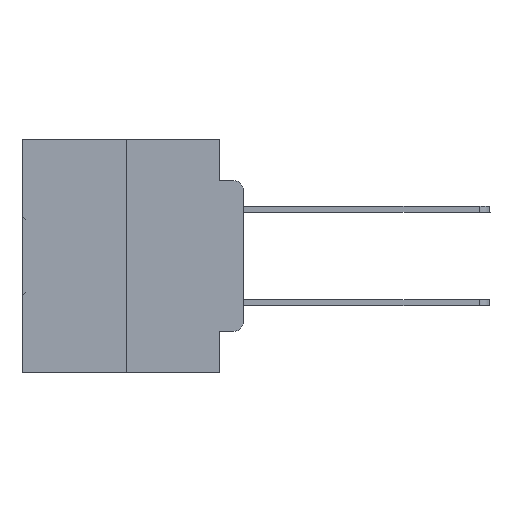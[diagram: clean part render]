
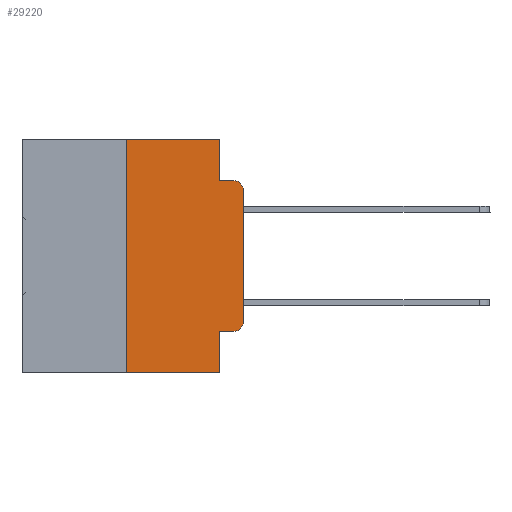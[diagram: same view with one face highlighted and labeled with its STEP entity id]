
A CAD part, left-side view. The second image highlights one B-rep face of the part: STEP entity #29220.
In plain terms, the highlighted planar face has unit normal (-1, 0, 0).
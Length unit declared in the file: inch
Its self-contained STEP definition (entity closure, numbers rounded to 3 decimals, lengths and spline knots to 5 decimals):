
#249 = DIRECTION ( 'NONE',  ( 0., -1., 0. ) ) ;
#351 = ORIENTED_EDGE ( 'NONE', *, *, #30464, .T. ) ;
#605 = AXIS2_PLACEMENT_3D ( 'NONE', #6944, #9692, #12454 ) ;
#1002 = VERTEX_POINT ( 'NONE', #11561 ) ;
#1033 = LINE ( 'NONE', #9492, #12632 ) ;
#1178 = LINE ( 'NONE', #33012, #11439 ) ;
#1340 = DIRECTION ( 'NONE',  ( 0., 0., -1. ) ) ;
#1547 = CARTESIAN_POINT ( 'NONE',  ( 0., 0.051, -0.4115 ) ) ;
#1676 = DIRECTION ( 'NONE',  ( 0., -1., 0. ) ) ;
#2059 = VERTEX_POINT ( 'NONE', #20706 ) ;
#2615 = LINE ( 'NONE', #14983, #34724 ) ;
#2622 = EDGE_CURVE ( 'NONE', #31842, #2059, #31884, .T. ) ;
#2749 = VECTOR ( 'NONE', #5492, 39.37008 ) ;
#3475 = EDGE_CURVE ( 'NONE', #24998, #34093, #28788, .T. ) ;
#4297 = LINE ( 'NONE', #15519, #11556 ) ;
#4590 = ORIENTED_EDGE ( 'NONE', *, *, #22030, .T. ) ;
#4610 = EDGE_CURVE ( 'NONE', #29883, #33204, #4297, .T. ) ;
#4845 = CIRCLE ( 'NONE', #26368, 0.02 ) ;
#4885 = CARTESIAN_POINT ( 'NONE',  ( 0., 0., -0.3915 ) ) ;
#5492 = DIRECTION ( 'NONE',  ( 0., -1., 0. ) ) ;
#6262 = DIRECTION ( 'NONE',  ( -1., 0., 0. ) ) ;
#6421 = LINE ( 'NONE', #1547, #15430 ) ;
#6808 = PLANE ( 'NONE',  #605 ) ;
#6880 = CARTESIAN_POINT ( 'NONE',  ( 0., 0.051, -0.4115 ) ) ;
#6944 = CARTESIAN_POINT ( 'NONE',  ( 0., 0.473, 0. ) ) ;
#7432 = VECTOR ( 'NONE', #32172, 39.37008 ) ;
#8366 = ORIENTED_EDGE ( 'NONE', *, *, #4610, .F. ) ;
#8964 = VERTEX_POINT ( 'NONE', #4885 ) ;
#9171 = EDGE_CURVE ( 'NONE', #1002, #15084, #2615, .T. ) ;
#9340 = AXIS2_PLACEMENT_3D ( 'NONE', #24849, #25208, #13945 ) ;
#9492 = CARTESIAN_POINT ( 'NONE',  ( 0., 0., 0. ) ) ;
#9564 = ORIENTED_EDGE ( 'NONE', *, *, #33394, .T. ) ;
#9692 = DIRECTION ( 'NONE',  ( 1., 0., 0. ) ) ;
#10059 = LINE ( 'NONE', #35440, #2749 ) ;
#10999 = FACE_OUTER_BOUND ( 'NONE', #34193, .T. ) ;
#11380 = CARTESIAN_POINT ( 'NONE',  ( 0., 0.051, -0.0885 ) ) ;
#11439 = VECTOR ( 'NONE', #19059, 39.37008 ) ;
#11458 = CARTESIAN_POINT ( 'NONE',  ( 0., 0., -0.1085 ) ) ;
#11556 = VECTOR ( 'NONE', #23700, 39.37008 ) ;
#11561 = CARTESIAN_POINT ( 'NONE',  ( 0., 0.051, 0. ) ) ;
#11948 = EDGE_CURVE ( 'NONE', #33204, #1002, #1178, .T. ) ;
#12454 = DIRECTION ( 'NONE',  ( 0., 0., -1. ) ) ;
#12632 = VECTOR ( 'NONE', #31258, 39.37008 ) ;
#13011 = CARTESIAN_POINT ( 'NONE',  ( 0., 0.051, 0. ) ) ;
#13180 = CARTESIAN_POINT ( 'NONE',  ( 0., 0.051, -0.0885 ) ) ;
#13945 = DIRECTION ( 'NONE',  ( 0., 0., -1. ) ) ;
#14983 = CARTESIAN_POINT ( 'NONE',  ( 0., 0.051, 0. ) ) ;
#15073 = VERTEX_POINT ( 'NONE', #19464 ) ;
#15084 = VERTEX_POINT ( 'NONE', #11380 ) ;
#15430 = VECTOR ( 'NONE', #1676, 39.37008 ) ;
#15519 = CARTESIAN_POINT ( 'NONE',  ( 0., 0.25, 0. ) ) ;
#19059 = DIRECTION ( 'NONE',  ( 0., -1., 0. ) ) ;
#19402 = ORIENTED_EDGE ( 'NONE', *, *, #2622, .F. ) ;
#19464 = CARTESIAN_POINT ( 'NONE',  ( 0., 0.02, -0.4115 ) ) ;
#20470 = CARTESIAN_POINT ( 'NONE',  ( 0., 0.25, -0.5 ) ) ;
#20706 = CARTESIAN_POINT ( 'NONE',  ( 0., 0.051, -0.5 ) ) ;
#22030 = EDGE_CURVE ( 'NONE', #31842, #15073, #6421, .T. ) ;
#23700 = DIRECTION ( 'NONE',  ( 0., 0., 1. ) ) ;
#24650 = VECTOR ( 'NONE', #249, 39.37008 ) ;
#24849 = CARTESIAN_POINT ( 'NONE',  ( 0., 0.02, -0.1085 ) ) ;
#24998 = VERTEX_POINT ( 'NONE', #11458 ) ;
#25208 = DIRECTION ( 'NONE',  ( -1., 0., 0. ) ) ;
#25355 = DIRECTION ( 'NONE',  ( 0., 0., -1. ) ) ;
#26368 = AXIS2_PLACEMENT_3D ( 'NONE', #28036, #6262, #25355 ) ;
#28036 = CARTESIAN_POINT ( 'NONE',  ( 0., 0.02, -0.3915 ) ) ;
#28788 = CIRCLE ( 'NONE', #9340, 0.02 ) ;
#28814 = ORIENTED_EDGE ( 'NONE', *, *, #32697, .T. ) ;
#28861 = EDGE_CURVE ( 'NONE', #15084, #34093, #32898, .T. ) ;
#29220 = ADVANCED_FACE ( 'NONE', ( #10999 ), #6808, .F. ) ;
#29883 = VERTEX_POINT ( 'NONE', #20470 ) ;
#29898 = ORIENTED_EDGE ( 'NONE', *, *, #28861, .F. ) ;
#30464 = EDGE_CURVE ( 'NONE', #8964, #24998, #1033, .T. ) ;
#31258 = DIRECTION ( 'NONE',  ( 0., 0., 1. ) ) ;
#31802 = ORIENTED_EDGE ( 'NONE', *, *, #3475, .T. ) ;
#31842 = VERTEX_POINT ( 'NONE', #6880 ) ;
#31884 = LINE ( 'NONE', #13011, #7432 ) ;
#32172 = DIRECTION ( 'NONE',  ( 0., 0., -1. ) ) ;
#32353 = CARTESIAN_POINT ( 'NONE',  ( 0., 0.02, -0.0885 ) ) ;
#32549 = CARTESIAN_POINT ( 'NONE',  ( 0., 0.25, 0. ) ) ;
#32697 = EDGE_CURVE ( 'NONE', #29883, #2059, #10059, .T. ) ;
#32898 = LINE ( 'NONE', #13180, #24650 ) ;
#33012 = CARTESIAN_POINT ( 'NONE',  ( 0., 0.473, 0. ) ) ;
#33204 = VERTEX_POINT ( 'NONE', #32549 ) ;
#33394 = EDGE_CURVE ( 'NONE', #15073, #8964, #4845, .T. ) ;
#34093 = VERTEX_POINT ( 'NONE', #32353 ) ;
#34101 = ORIENTED_EDGE ( 'NONE', *, *, #11948, .F. ) ;
#34193 = EDGE_LOOP ( 'NONE', ( #351, #31802, #29898, #34241, #34101, #8366, #28814, #19402, #4590, #9564 ) ) ;
#34241 = ORIENTED_EDGE ( 'NONE', *, *, #9171, .F. ) ;
#34724 = VECTOR ( 'NONE', #1340, 39.37008 ) ;
#35440 = CARTESIAN_POINT ( 'NONE',  ( 0., 0.473, -0.5 ) ) ;
